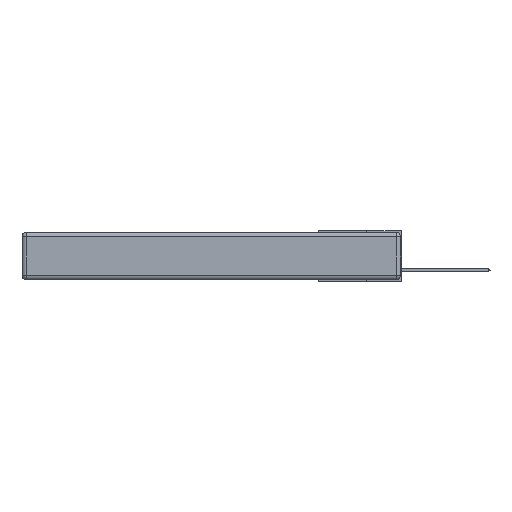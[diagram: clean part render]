
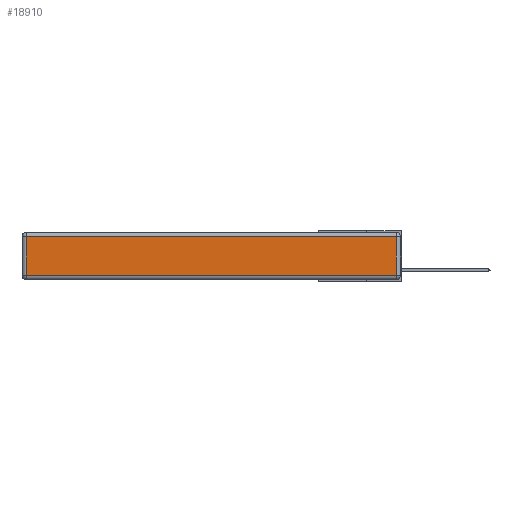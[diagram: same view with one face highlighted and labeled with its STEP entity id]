
A CAD part, left-side view. The second image highlights one B-rep face of the part: STEP entity #18910.
In plain terms, the highlighted planar face has unit normal (-1, 0, 0).
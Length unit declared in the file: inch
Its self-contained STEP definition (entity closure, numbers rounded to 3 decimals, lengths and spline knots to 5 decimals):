
#1238 = CARTESIAN_POINT ( 'NONE',  ( 0., 2.75, -0.03 ) ) ;
#1569 = EDGE_CURVE ( 'NONE', #14507, #11532, #20932, .T. ) ;
#1682 = EDGE_CURVE ( 'NONE', #11532, #4209, #2062, .T. ) ;
#2062 = LINE ( 'NONE', #1238, #13079 ) ;
#2512 = LINE ( 'NONE', #17459, #14862 ) ;
#2559 = DIRECTION ( 'NONE',  ( 0., 0., 1. ) ) ;
#3313 = CARTESIAN_POINT ( 'NONE',  ( 0., 0.03, -0.313 ) ) ;
#3317 = CARTESIAN_POINT ( 'NONE',  ( 0., 2.72, -0.313 ) ) ;
#3388 = FACE_OUTER_BOUND ( 'NONE', #5490, .T. ) ;
#4209 = VERTEX_POINT ( 'NONE', #21400 ) ;
#4566 = CARTESIAN_POINT ( 'NONE',  ( 0., 0.03, -0.343 ) ) ;
#4897 = VECTOR ( 'NONE', #10977, 39.37008 ) ;
#5490 = EDGE_LOOP ( 'NONE', ( #9990, #17362, #10826, #12934 ) ) ;
#5862 = CARTESIAN_POINT ( 'NONE',  ( 0., 2.72, -0.343 ) ) ;
#7298 = CARTESIAN_POINT ( 'NONE',  ( 0., 0., -0.343 ) ) ;
#7413 = CARTESIAN_POINT ( 'NONE',  ( 0., 0.03, -0.03 ) ) ;
#9000 = DIRECTION ( 'NONE',  ( 0., 0., 1. ) ) ;
#9492 = VERTEX_POINT ( 'NONE', #3317 ) ;
#9990 = ORIENTED_EDGE ( 'NONE', *, *, #20540, .T. ) ;
#10826 = ORIENTED_EDGE ( 'NONE', *, *, #1682, .T. ) ;
#10977 = DIRECTION ( 'NONE',  ( 0., 0., -1. ) ) ;
#11532 = VERTEX_POINT ( 'NONE', #7413 ) ;
#12515 = PLANE ( 'NONE',  #15073 ) ;
#12934 = ORIENTED_EDGE ( 'NONE', *, *, #20428, .T. ) ;
#13079 = VECTOR ( 'NONE', #16651, 39.37008 ) ;
#14399 = VECTOR ( 'NONE', #2559, 39.37008 ) ;
#14507 = VERTEX_POINT ( 'NONE', #3313 ) ;
#14576 = LINE ( 'NONE', #5862, #4897 ) ;
#14862 = VECTOR ( 'NONE', #20820, 39.37008 ) ;
#15073 = AXIS2_PLACEMENT_3D ( 'NONE', #7298, #17231, #9000 ) ;
#16651 = DIRECTION ( 'NONE',  ( 0., 1., 0. ) ) ;
#17231 = DIRECTION ( 'NONE',  ( -1., 0., 0. ) ) ;
#17362 = ORIENTED_EDGE ( 'NONE', *, *, #1569, .T. ) ;
#17459 = CARTESIAN_POINT ( 'NONE',  ( 0., 0., -0.313 ) ) ;
#18910 = ADVANCED_FACE ( 'NONE', ( #3388 ), #12515, .T. ) ;
#20428 = EDGE_CURVE ( 'NONE', #4209, #9492, #14576, .T. ) ;
#20540 = EDGE_CURVE ( 'NONE', #9492, #14507, #2512, .T. ) ;
#20820 = DIRECTION ( 'NONE',  ( 0., -1., 0. ) ) ;
#20932 = LINE ( 'NONE', #4566, #14399 ) ;
#21400 = CARTESIAN_POINT ( 'NONE',  ( 0., 2.72, -0.03 ) ) ;
